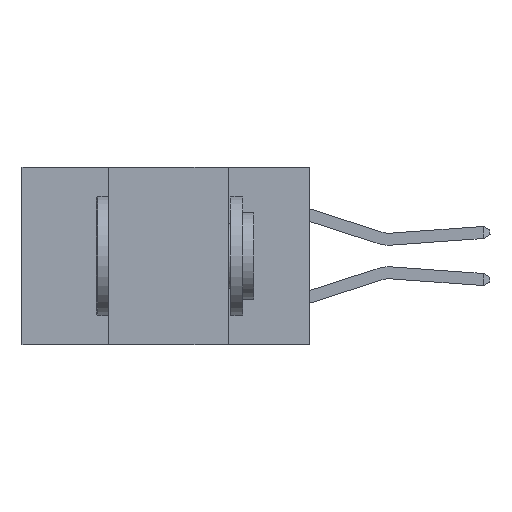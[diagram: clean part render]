
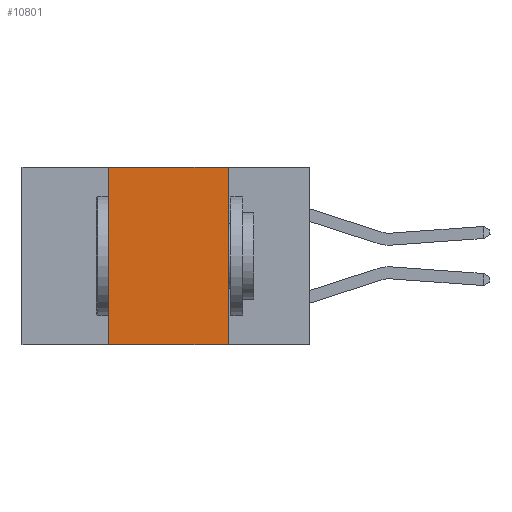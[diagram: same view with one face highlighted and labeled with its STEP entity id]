
A CAD part, left-side view. The second image highlights one B-rep face of the part: STEP entity #10801.
In plain terms, the highlighted planar face has unit normal (-1, 0, 0).
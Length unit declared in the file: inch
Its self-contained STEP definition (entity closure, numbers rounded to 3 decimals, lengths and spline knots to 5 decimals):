
#837 = VECTOR ( 'NONE', #4688, 39.37008 ) ;
#1431 = CARTESIAN_POINT ( 'NONE',  ( 0., 0.6, -0.37 ) ) ;
#1520 = DIRECTION ( 'NONE',  ( 1., 0., 0. ) ) ;
#1683 = ORIENTED_EDGE ( 'NONE', *, *, #10147, .F. ) ;
#1787 = VERTEX_POINT ( 'NONE', #11526 ) ;
#2860 = DIRECTION ( 'NONE',  ( 0., 0., -1. ) ) ;
#2968 = ORIENTED_EDGE ( 'NONE', *, *, #10776, .T. ) ;
#3789 = VERTEX_POINT ( 'NONE', #5354 ) ;
#4688 = DIRECTION ( 'NONE',  ( 0., 0., -1. ) ) ;
#4843 = EDGE_CURVE ( 'NONE', #7448, #1787, #15292, .T. ) ;
#5354 = CARTESIAN_POINT ( 'NONE',  ( 0., 0.42, -0.37 ) ) ;
#5415 = ORIENTED_EDGE ( 'NONE', *, *, #16766, .F. ) ;
#5500 = CARTESIAN_POINT ( 'NONE',  ( 0., 0.42, -0.37 ) ) ;
#6429 = AXIS2_PLACEMENT_3D ( 'NONE', #16203, #1520, #2860 ) ;
#6579 = LINE ( 'NONE', #5500, #16994 ) ;
#7448 = VERTEX_POINT ( 'NONE', #17482 ) ;
#7617 = CARTESIAN_POINT ( 'NONE',  ( 0., 0.17, -0.37 ) ) ;
#8901 = PLANE ( 'NONE',  #6429 ) ;
#10147 = EDGE_CURVE ( 'NONE', #3789, #7448, #6579, .T. ) ;
#10776 = EDGE_CURVE ( 'NONE', #3789, #12679, #13187, .T. ) ;
#10801 = ADVANCED_FACE ( 'NONE', ( #14448 ), #8901, .F. ) ;
#11526 = CARTESIAN_POINT ( 'NONE',  ( 0., 0.17, 0. ) ) ;
#11976 = ORIENTED_EDGE ( 'NONE', *, *, #4843, .F. ) ;
#12482 = EDGE_LOOP ( 'NONE', ( #5415, #11976, #1683, #2968 ) ) ;
#12530 = DIRECTION ( 'NONE',  ( 0., 0., 1. ) ) ;
#12621 = CARTESIAN_POINT ( 'NONE',  ( 0., 0.17, -0.37 ) ) ;
#12679 = VERTEX_POINT ( 'NONE', #12621 ) ;
#12980 = DIRECTION ( 'NONE',  ( 0., -1., 0. ) ) ;
#13187 = LINE ( 'NONE', #1431, #18243 ) ;
#13829 = DIRECTION ( 'NONE',  ( 0., -1., 0. ) ) ;
#13924 = CARTESIAN_POINT ( 'NONE',  ( 0., 0.6, 0. ) ) ;
#14448 = FACE_OUTER_BOUND ( 'NONE', #12482, .T. ) ;
#15006 = LINE ( 'NONE', #7617, #837 ) ;
#15292 = LINE ( 'NONE', #13924, #15517 ) ;
#15517 = VECTOR ( 'NONE', #13829, 39.37008 ) ;
#16203 = CARTESIAN_POINT ( 'NONE',  ( 0., 0.6, 0. ) ) ;
#16766 = EDGE_CURVE ( 'NONE', #1787, #12679, #15006, .T. ) ;
#16994 = VECTOR ( 'NONE', #12530, 39.37008 ) ;
#17482 = CARTESIAN_POINT ( 'NONE',  ( 0., 0.42, 0. ) ) ;
#18243 = VECTOR ( 'NONE', #12980, 39.37008 ) ;
